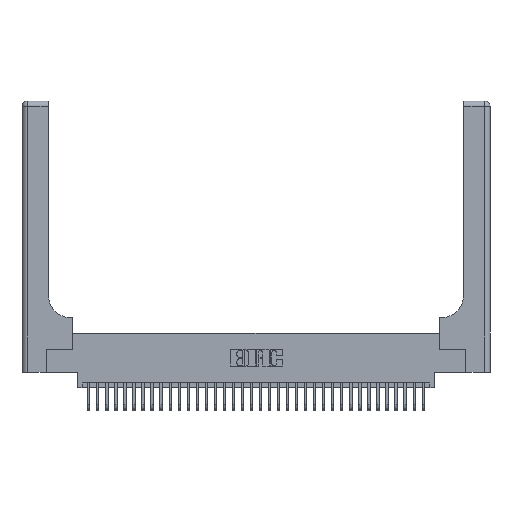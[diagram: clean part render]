
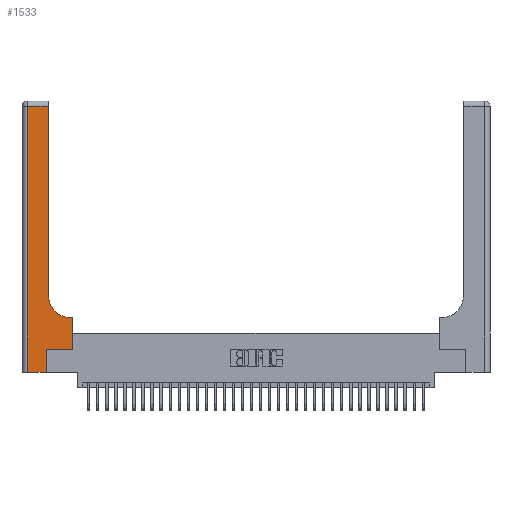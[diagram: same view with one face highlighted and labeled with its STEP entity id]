
A CAD part, top view. The second image highlights one B-rep face of the part: STEP entity #1533.
In plain terms, the highlighted planar face has unit normal (0, 0, 1).
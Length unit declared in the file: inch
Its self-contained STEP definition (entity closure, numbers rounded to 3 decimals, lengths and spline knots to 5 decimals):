
#201 = EDGE_CURVE ( 'NONE', #4039, #35663, #9659, .T. ) ;
#336 = DIRECTION ( 'NONE',  ( 0., 1., 0. ) ) ;
#860 = CARTESIAN_POINT ( 'NONE',  ( 0.269, 0., 0.37 ) ) ;
#1022 = VECTOR ( 'NONE', #16160, 39.37008 ) ;
#1296 = AXIS2_PLACEMENT_3D ( 'NONE', #21393, #14300, #31961 ) ;
#1368 = EDGE_CURVE ( 'NONE', #19349, #20846, #21846, .T. ) ;
#1533 = ADVANCED_FACE ( 'NONE', ( #17326 ), #27587, .F. ) ;
#1577 = EDGE_LOOP ( 'NONE', ( #24746, #4100, #23738, #30061, #32685, #20437, #19976, #16896, #18088 ) ) ;
#1582 = CARTESIAN_POINT ( 'NONE',  ( 0.269, 0.25, 0.37 ) ) ;
#4039 = VERTEX_POINT ( 'NONE', #19060 ) ;
#4100 = ORIENTED_EDGE ( 'NONE', *, *, #8561, .T. ) ;
#4156 = VERTEX_POINT ( 'NONE', #30752 ) ;
#4473 = LINE ( 'NONE', #14458, #28790 ) ;
#4589 = VECTOR ( 'NONE', #26610, 39.37008 ) ;
#5522 = VERTEX_POINT ( 'NONE', #27517 ) ;
#7865 = EDGE_CURVE ( 'NONE', #5522, #13212, #32491, .T. ) ;
#8561 = EDGE_CURVE ( 'NONE', #30011, #4156, #36061, .T. ) ;
#9240 = DIRECTION ( 'NONE',  ( 0., 1., 0. ) ) ;
#9659 = CIRCLE ( 'NONE', #20562, 0.25 ) ;
#9854 = CARTESIAN_POINT ( 'NONE',  ( 0.5415, 0.85, 0.37 ) ) ;
#9857 = CARTESIAN_POINT ( 'NONE',  ( 0., 2.94, 0.37 ) ) ;
#9994 = DIRECTION ( 'NONE',  ( 0., 0., -1. ) ) ;
#10417 = VECTOR ( 'NONE', #13676, 39.37008 ) ;
#10990 = CARTESIAN_POINT ( 'NONE',  ( 0.06, 3., 0.37 ) ) ;
#13027 = DIRECTION ( 'NONE',  ( 1., 0., 0. ) ) ;
#13212 = VERTEX_POINT ( 'NONE', #29964 ) ;
#13676 = DIRECTION ( 'NONE',  ( 0., -1., 0. ) ) ;
#14300 = DIRECTION ( 'NONE',  ( 0., 0., -1. ) ) ;
#14458 = CARTESIAN_POINT ( 'NONE',  ( 0.2915, 3., 0.37 ) ) ;
#16160 = DIRECTION ( 'NONE',  ( 1., 0., 0. ) ) ;
#16896 = ORIENTED_EDGE ( 'NONE', *, *, #25962, .T. ) ;
#16981 = EDGE_CURVE ( 'NONE', #4156, #5522, #26580, .T. ) ;
#17326 = FACE_OUTER_BOUND ( 'NONE', #1577, .T. ) ;
#18088 = ORIENTED_EDGE ( 'NONE', *, *, #201, .T. ) ;
#18626 = LINE ( 'NONE', #32693, #24921 ) ;
#18728 = EDGE_CURVE ( 'NONE', #35663, #30011, #4473, .T. ) ;
#19060 = CARTESIAN_POINT ( 'NONE',  ( 0.5415, 0.6, 0.37 ) ) ;
#19349 = VERTEX_POINT ( 'NONE', #30074 ) ;
#19379 = LINE ( 'NONE', #23278, #22988 ) ;
#19976 = ORIENTED_EDGE ( 'NONE', *, *, #28014, .T. ) ;
#20346 = CARTESIAN_POINT ( 'NONE',  ( 0., 0., 0.37 ) ) ;
#20437 = ORIENTED_EDGE ( 'NONE', *, *, #1368, .T. ) ;
#20562 = AXIS2_PLACEMENT_3D ( 'NONE', #9854, #9994, #13027 ) ;
#20846 = VERTEX_POINT ( 'NONE', #35224 ) ;
#20951 = DIRECTION ( 'NONE',  ( 0., 1., 0. ) ) ;
#21120 = VERTEX_POINT ( 'NONE', #36488 ) ;
#21393 = CARTESIAN_POINT ( 'NONE',  ( 0., 3., 0.37 ) ) ;
#21708 = VECTOR ( 'NONE', #9240, 39.37008 ) ;
#21846 = LINE ( 'NONE', #1582, #1022 ) ;
#22988 = VECTOR ( 'NONE', #20951, 39.37008 ) ;
#23278 = CARTESIAN_POINT ( 'NONE',  ( 0.5585, 0.25, 0.37 ) ) ;
#23738 = ORIENTED_EDGE ( 'NONE', *, *, #16981, .T. ) ;
#23836 = DIRECTION ( 'NONE',  ( -1., 0., 0. ) ) ;
#24376 = CARTESIAN_POINT ( 'NONE',  ( 0.2915, 0.85, 0.37 ) ) ;
#24746 = ORIENTED_EDGE ( 'NONE', *, *, #18728, .T. ) ;
#24921 = VECTOR ( 'NONE', #26531, 39.37008 ) ;
#25962 = EDGE_CURVE ( 'NONE', #21120, #4039, #18626, .T. ) ;
#26531 = DIRECTION ( 'NONE',  ( -1., 0., 0. ) ) ;
#26580 = LINE ( 'NONE', #10990, #10417 ) ;
#26610 = DIRECTION ( 'NONE',  ( 1., 0., 0. ) ) ;
#26739 = EDGE_CURVE ( 'NONE', #13212, #19349, #34740, .T. ) ;
#27517 = CARTESIAN_POINT ( 'NONE',  ( 0.06, 0., 0.37 ) ) ;
#27587 = PLANE ( 'NONE',  #1296 ) ;
#28014 = EDGE_CURVE ( 'NONE', #20846, #21120, #19379, .T. ) ;
#28790 = VECTOR ( 'NONE', #336, 39.37008 ) ;
#29964 = CARTESIAN_POINT ( 'NONE',  ( 0.269, 0., 0.37 ) ) ;
#30011 = VERTEX_POINT ( 'NONE', #35605 ) ;
#30061 = ORIENTED_EDGE ( 'NONE', *, *, #7865, .T. ) ;
#30074 = CARTESIAN_POINT ( 'NONE',  ( 0.269, 0.25, 0.37 ) ) ;
#30752 = CARTESIAN_POINT ( 'NONE',  ( 0.06, 2.94, 0.37 ) ) ;
#31961 = DIRECTION ( 'NONE',  ( -1., 0., 0. ) ) ;
#32491 = LINE ( 'NONE', #20346, #4589 ) ;
#32685 = ORIENTED_EDGE ( 'NONE', *, *, #26739, .T. ) ;
#32693 = CARTESIAN_POINT ( 'NONE',  ( 0.2915, 0.6, 0.37 ) ) ;
#34740 = LINE ( 'NONE', #860, #21708 ) ;
#35121 = VECTOR ( 'NONE', #23836, 39.37008 ) ;
#35224 = CARTESIAN_POINT ( 'NONE',  ( 0.5585, 0.25, 0.37 ) ) ;
#35605 = CARTESIAN_POINT ( 'NONE',  ( 0.2915, 2.94, 0.37 ) ) ;
#35663 = VERTEX_POINT ( 'NONE', #24376 ) ;
#36061 = LINE ( 'NONE', #9857, #35121 ) ;
#36488 = CARTESIAN_POINT ( 'NONE',  ( 0.5585, 0.6, 0.37 ) ) ;
